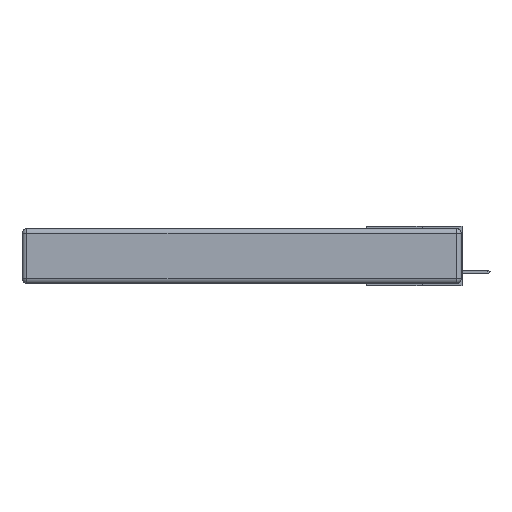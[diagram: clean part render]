
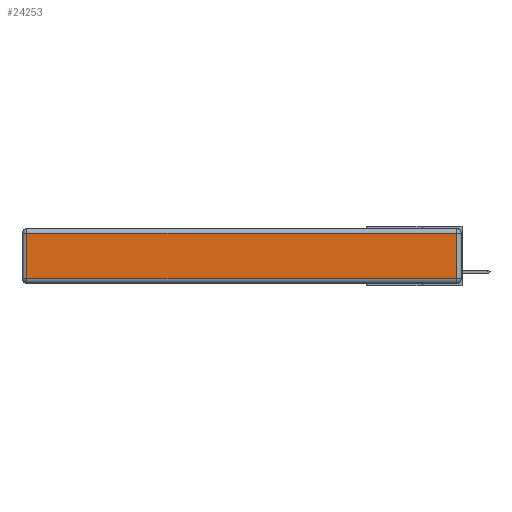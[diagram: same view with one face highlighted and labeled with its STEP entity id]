
A CAD part, left-side view. The second image highlights one B-rep face of the part: STEP entity #24253.
In plain terms, the highlighted planar face has unit normal (-1, 0, 0).
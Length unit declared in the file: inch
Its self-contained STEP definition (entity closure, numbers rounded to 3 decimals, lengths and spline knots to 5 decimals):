
#149 = CARTESIAN_POINT ( 'NONE',  ( 0., 2.72, -0.313 ) ) ;
#302 = DIRECTION ( 'NONE',  ( 0., -1., 0. ) ) ;
#973 = EDGE_CURVE ( 'NONE', #14604, #13259, #11524, .T. ) ;
#4043 = DIRECTION ( 'NONE',  ( -1., 0., 0. ) ) ;
#4134 = VERTEX_POINT ( 'NONE', #21564 ) ;
#4284 = CARTESIAN_POINT ( 'NONE',  ( 0., 2.75, -0.03 ) ) ;
#4355 = VECTOR ( 'NONE', #10760, 39.37008 ) ;
#5354 = EDGE_CURVE ( 'NONE', #4134, #14604, #18572, .T. ) ;
#6530 = CARTESIAN_POINT ( 'NONE',  ( 0., 2.72, -0.343 ) ) ;
#6688 = CARTESIAN_POINT ( 'NONE',  ( 0., 0.03, -0.343 ) ) ;
#6782 = VECTOR ( 'NONE', #15228, 39.37008 ) ;
#6840 = ORIENTED_EDGE ( 'NONE', *, *, #20947, .T. ) ;
#7923 = VERTEX_POINT ( 'NONE', #27824 ) ;
#10760 = DIRECTION ( 'NONE',  ( 0., 1., 0. ) ) ;
#11524 = LINE ( 'NONE', #21783, #16608 ) ;
#11620 = EDGE_LOOP ( 'NONE', ( #27088, #6840, #19559, #18342 ) ) ;
#11906 = EDGE_CURVE ( 'NONE', #7923, #4134, #13766, .T. ) ;
#11946 = DIRECTION ( 'NONE',  ( 0., 0., 1. ) ) ;
#13259 = VERTEX_POINT ( 'NONE', #19748 ) ;
#13766 = LINE ( 'NONE', #4284, #4355 ) ;
#14604 = VERTEX_POINT ( 'NONE', #149 ) ;
#15228 = DIRECTION ( 'NONE',  ( 0., 0., -1. ) ) ;
#16608 = VECTOR ( 'NONE', #302, 39.37008 ) ;
#16936 = DIRECTION ( 'NONE',  ( 0., 0., 1. ) ) ;
#17622 = AXIS2_PLACEMENT_3D ( 'NONE', #25189, #4043, #16936 ) ;
#18342 = ORIENTED_EDGE ( 'NONE', *, *, #5354, .T. ) ;
#18572 = LINE ( 'NONE', #6530, #6782 ) ;
#18988 = PLANE ( 'NONE',  #17622 ) ;
#19145 = VECTOR ( 'NONE', #11946, 39.37008 ) ;
#19559 = ORIENTED_EDGE ( 'NONE', *, *, #11906, .T. ) ;
#19748 = CARTESIAN_POINT ( 'NONE',  ( 0., 0.03, -0.313 ) ) ;
#20947 = EDGE_CURVE ( 'NONE', #13259, #7923, #22176, .T. ) ;
#21564 = CARTESIAN_POINT ( 'NONE',  ( 0., 2.72, -0.03 ) ) ;
#21783 = CARTESIAN_POINT ( 'NONE',  ( 0., 0., -0.313 ) ) ;
#22176 = LINE ( 'NONE', #6688, #19145 ) ;
#24253 = ADVANCED_FACE ( 'NONE', ( #27708 ), #18988, .T. ) ;
#25189 = CARTESIAN_POINT ( 'NONE',  ( 0., 0., -0.343 ) ) ;
#27088 = ORIENTED_EDGE ( 'NONE', *, *, #973, .T. ) ;
#27708 = FACE_OUTER_BOUND ( 'NONE', #11620, .T. ) ;
#27824 = CARTESIAN_POINT ( 'NONE',  ( 0., 0.03, -0.03 ) ) ;
